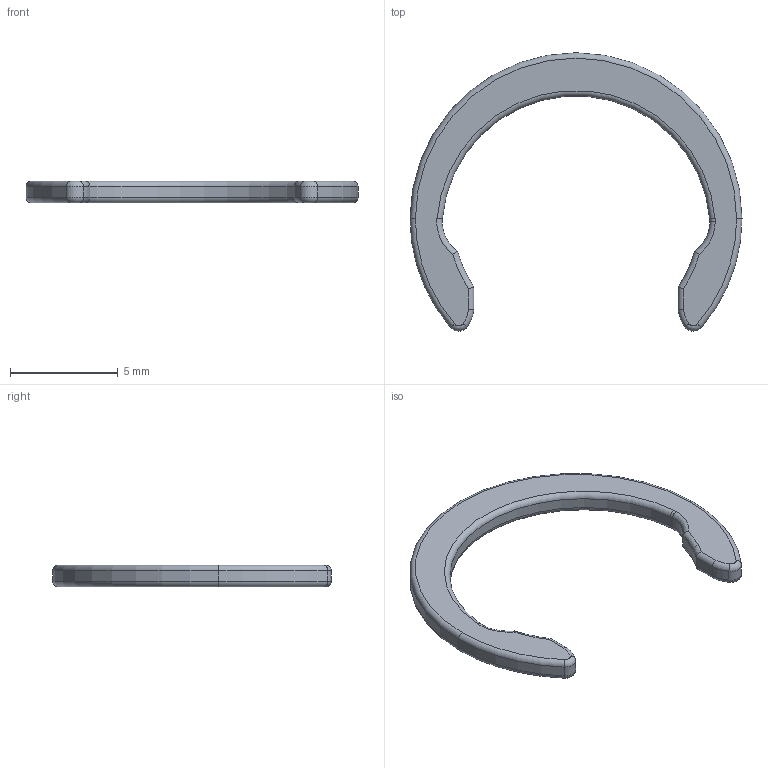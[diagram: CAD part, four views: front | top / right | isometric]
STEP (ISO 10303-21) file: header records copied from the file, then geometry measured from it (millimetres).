
FILE_DESCRIPTION (( 'STEP AP214' ), '1' );
FILE_NAME ('90119A102_Low-Clearance External Retaining Rings.STEP', '2025-05-18T10:37:41', ( '' ), ( '' ), 'SwSTEP 2.0', 'SolidWorks 2024', '' );
FILE_SCHEMA (( 'AUTOMOTIVE_DESIGN' ));
Length unit declared in the file: millimetre
Products named in the file (1): 90119A102_Low-Clearance External Retaining Rings_90119A102
Bounding box: 15.4 x 12.91 x 1 mm (x, y, z)
Volume: 55.6 mm3; surface area: 166.9 mm2
Topology: 1 solids, 1 shells, 47 faces, 107 edges, 62 vertices
Faces by surface type: torus 26, cylinder 17, plane 4
Entity records: 1388 total; most frequent: CARTESIAN_POINT 277, DIRECTION 263, ORIENTED_EDGE 214, AXIS2_PLACEMENT_3D 120, EDGE_CURVE 107, CIRCLE 72, VERTEX_POINT 62, ADVANCED_FACE 47
